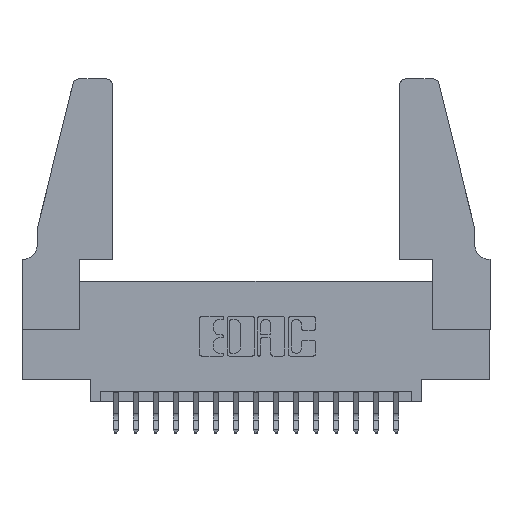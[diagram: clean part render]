
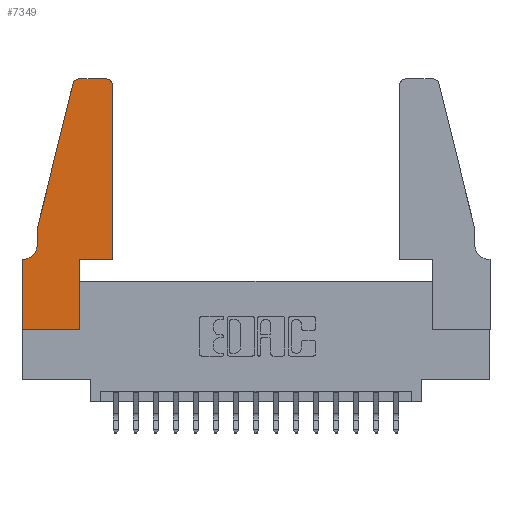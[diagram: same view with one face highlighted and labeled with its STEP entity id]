
A CAD part, top view. The second image highlights one B-rep face of the part: STEP entity #7349.
In plain terms, the highlighted planar face has unit normal (0, 0, 1).
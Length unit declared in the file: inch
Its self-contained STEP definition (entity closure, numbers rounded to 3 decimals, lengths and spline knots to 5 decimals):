
#104 = DIRECTION ( 'NONE',  ( 0., 0., 1. ) ) ;
#455 = VECTOR ( 'NONE', #6482, 39.37008 ) ;
#690 = ORIENTED_EDGE ( 'NONE', *, *, #16644, .T. ) ;
#772 = ORIENTED_EDGE ( 'NONE', *, *, #14668, .T. ) ;
#830 = CARTESIAN_POINT ( 'NONE',  ( 0.0055, 0.35, 0.37 ) ) ;
#983 = CARTESIAN_POINT ( 'NONE',  ( 0.4505, 0.35, 0.37 ) ) ;
#1338 = CIRCLE ( 'NONE', #2276, 0.07 ) ;
#1379 = EDGE_CURVE ( 'NONE', #8854, #14254, #16384, .T. ) ;
#1571 = ORIENTED_EDGE ( 'NONE', *, *, #17918, .T. ) ;
#1724 = VERTEX_POINT ( 'NONE', #7770 ) ;
#1811 = EDGE_CURVE ( 'NONE', #17260, #10130, #5855, .T. ) ;
#1948 = VERTEX_POINT ( 'NONE', #7112 ) ;
#2093 = ORIENTED_EDGE ( 'NONE', *, *, #16636, .T. ) ;
#2276 = AXIS2_PLACEMENT_3D ( 'NONE', #12101, #3801, #13503 ) ;
#2937 = PLANE ( 'NONE',  #3319 ) ;
#3049 = VECTOR ( 'NONE', #5222, 39.37008 ) ;
#3319 = AXIS2_PLACEMENT_3D ( 'NONE', #15407, #104, #9956 ) ;
#3765 = CARTESIAN_POINT ( 'NONE',  ( 0.4505, 1.22, 0.37 ) ) ;
#3801 = DIRECTION ( 'NONE',  ( 0., 0., -1. ) ) ;
#3812 = LINE ( 'NONE', #16098, #455 ) ;
#4005 = AXIS2_PLACEMENT_3D ( 'NONE', #9490, #12695, #9902 ) ;
#4219 = DIRECTION ( 'NONE',  ( 1., 0., 0. ) ) ;
#4436 = LINE ( 'NONE', #5129, #11800 ) ;
#4560 = EDGE_CURVE ( 'NONE', #9600, #8854, #17265, .T. ) ;
#4595 = VECTOR ( 'NONE', #16410, 39.37008 ) ;
#4691 = ORIENTED_EDGE ( 'NONE', *, *, #4560, .T. ) ;
#5129 = CARTESIAN_POINT ( 'NONE',  ( 0.2605, 1.25, 0.37 ) ) ;
#5222 = DIRECTION ( 'NONE',  ( -0.239, -0.971, 0. ) ) ;
#5241 = VECTOR ( 'NONE', #15109, 39.37008 ) ;
#5321 = EDGE_CURVE ( 'NONE', #1724, #17935, #9797, .T. ) ;
#5440 = DIRECTION ( 'NONE',  ( 0., 0., 1. ) ) ;
#5737 = ORIENTED_EDGE ( 'NONE', *, *, #5321, .T. ) ;
#5855 = CIRCLE ( 'NONE', #4005, 0.03 ) ;
#6482 = DIRECTION ( 'NONE',  ( 0., -1., 0. ) ) ;
#6728 = CARTESIAN_POINT ( 'NONE',  ( 0.0755, 0.5, 0.37 ) ) ;
#6976 = ORIENTED_EDGE ( 'NONE', *, *, #14281, .T. ) ;
#7112 = CARTESIAN_POINT ( 'NONE',  ( 0., 0., 0.37 ) ) ;
#7349 = ADVANCED_FACE ( 'NONE', ( #13164 ), #2937, .T. ) ;
#7633 = VERTEX_POINT ( 'NONE', #9215 ) ;
#7647 = DIRECTION ( 'NONE',  ( 0., -1., 0. ) ) ;
#7649 = EDGE_CURVE ( 'NONE', #7633, #1948, #3812, .T. ) ;
#7770 = CARTESIAN_POINT ( 'NONE',  ( 0.2865, 0., 0.37 ) ) ;
#7967 = CARTESIAN_POINT ( 'NONE',  ( 0.4205, 1.25, 0.37 ) ) ;
#8000 = CARTESIAN_POINT ( 'NONE',  ( 0.0755, 0.5, 0.37 ) ) ;
#8075 = CARTESIAN_POINT ( 'NONE',  ( 0.2865, 0.35, 0.37 ) ) ;
#8101 = EDGE_CURVE ( 'NONE', #1948, #1724, #8192, .T. ) ;
#8192 = LINE ( 'NONE', #15952, #15077 ) ;
#8291 = CARTESIAN_POINT ( 'NONE',  ( 0.25487, 1.22718, 0.37 ) ) ;
#8292 = LINE ( 'NONE', #17624, #4595 ) ;
#8385 = ORIENTED_EDGE ( 'NONE', *, *, #1811, .T. ) ;
#8418 = ORIENTED_EDGE ( 'NONE', *, *, #7649, .T. ) ;
#8636 = EDGE_LOOP ( 'NONE', ( #772, #2093, #4691, #10306, #15851, #690, #8418, #9243, #5737, #6976, #1571, #8385 ) ) ;
#8753 = CARTESIAN_POINT ( 'NONE',  ( 0.0755, 0.5, 0.37 ) ) ;
#8854 = VERTEX_POINT ( 'NONE', #6728 ) ;
#9125 = DIRECTION ( 'NONE',  ( 1., 0., 0. ) ) ;
#9215 = CARTESIAN_POINT ( 'NONE',  ( 0., 0.35, 0.37 ) ) ;
#9237 = CARTESIAN_POINT ( 'NONE',  ( 0.4505, 0.35, 0.37 ) ) ;
#9243 = ORIENTED_EDGE ( 'NONE', *, *, #8101, .T. ) ;
#9347 = VECTOR ( 'NONE', #10803, 39.37008 ) ;
#9409 = VERTEX_POINT ( 'NONE', #830 ) ;
#9490 = CARTESIAN_POINT ( 'NONE',  ( 0.4205, 1.22, 0.37 ) ) ;
#9600 = VERTEX_POINT ( 'NONE', #8291 ) ;
#9682 = CARTESIAN_POINT ( 'NONE',  ( 0.0755, 0.42, 0.37 ) ) ;
#9797 = LINE ( 'NONE', #17715, #5241 ) ;
#9902 = DIRECTION ( 'NONE',  ( 1., 0., 0. ) ) ;
#9956 = DIRECTION ( 'NONE',  ( 1., 0., 0. ) ) ;
#10130 = VERTEX_POINT ( 'NONE', #7967 ) ;
#10306 = ORIENTED_EDGE ( 'NONE', *, *, #1379, .T. ) ;
#10540 = VECTOR ( 'NONE', #4219, 39.37008 ) ;
#10803 = DIRECTION ( 'NONE',  ( 0., 1., 0. ) ) ;
#11335 = CARTESIAN_POINT ( 'NONE',  ( 0.284, 1.25, 0.37 ) ) ;
#11800 = VECTOR ( 'NONE', #14768, 39.37008 ) ;
#11899 = AXIS2_PLACEMENT_3D ( 'NONE', #13710, #5440, #15067 ) ;
#12101 = CARTESIAN_POINT ( 'NONE',  ( 0.0055, 0.42, 0.37 ) ) ;
#12138 = LINE ( 'NONE', #983, #9347 ) ;
#12695 = DIRECTION ( 'NONE',  ( 0., 0., 1. ) ) ;
#13164 = FACE_OUTER_BOUND ( 'NONE', #8636, .T. ) ;
#13483 = EDGE_CURVE ( 'NONE', #14254, #9409, #1338, .T. ) ;
#13503 = DIRECTION ( 'NONE',  ( -1., 0., 0. ) ) ;
#13710 = CARTESIAN_POINT ( 'NONE',  ( 0.284, 1.22, 0.37 ) ) ;
#13904 = CARTESIAN_POINT ( 'NONE',  ( 0.4505, 0.35, 0.37 ) ) ;
#14254 = VERTEX_POINT ( 'NONE', #9682 ) ;
#14281 = EDGE_CURVE ( 'NONE', #17935, #15205, #17737, .T. ) ;
#14668 = EDGE_CURVE ( 'NONE', #10130, #14958, #4436, .T. ) ;
#14768 = DIRECTION ( 'NONE',  ( -1., 0., 0. ) ) ;
#14958 = VERTEX_POINT ( 'NONE', #11335 ) ;
#15067 = DIRECTION ( 'NONE',  ( 1., 0., 0. ) ) ;
#15077 = VECTOR ( 'NONE', #9125, 39.37008 ) ;
#15109 = DIRECTION ( 'NONE',  ( 0., 1., 0. ) ) ;
#15205 = VERTEX_POINT ( 'NONE', #9237 ) ;
#15407 = CARTESIAN_POINT ( 'NONE',  ( 0., 0.35, 0.37 ) ) ;
#15562 = VECTOR ( 'NONE', #7647, 39.37008 ) ;
#15598 = CIRCLE ( 'NONE', #11899, 0.03 ) ;
#15851 = ORIENTED_EDGE ( 'NONE', *, *, #13483, .T. ) ;
#15952 = CARTESIAN_POINT ( 'NONE',  ( 0., 0., 0.37 ) ) ;
#16098 = CARTESIAN_POINT ( 'NONE',  ( 0., 0., 0.37 ) ) ;
#16384 = LINE ( 'NONE', #8753, #15562 ) ;
#16410 = DIRECTION ( 'NONE',  ( -1., 0., 0. ) ) ;
#16636 = EDGE_CURVE ( 'NONE', #14958, #9600, #15598, .T. ) ;
#16644 = EDGE_CURVE ( 'NONE', #9409, #7633, #8292, .T. ) ;
#17260 = VERTEX_POINT ( 'NONE', #3765 ) ;
#17265 = LINE ( 'NONE', #8000, #3049 ) ;
#17624 = CARTESIAN_POINT ( 'NONE',  ( 0.0755, 0.35, 0.37 ) ) ;
#17715 = CARTESIAN_POINT ( 'NONE',  ( 0.2865, 0.35, 0.37 ) ) ;
#17737 = LINE ( 'NONE', #13904, #10540 ) ;
#17918 = EDGE_CURVE ( 'NONE', #15205, #17260, #12138, .T. ) ;
#17935 = VERTEX_POINT ( 'NONE', #8075 ) ;
